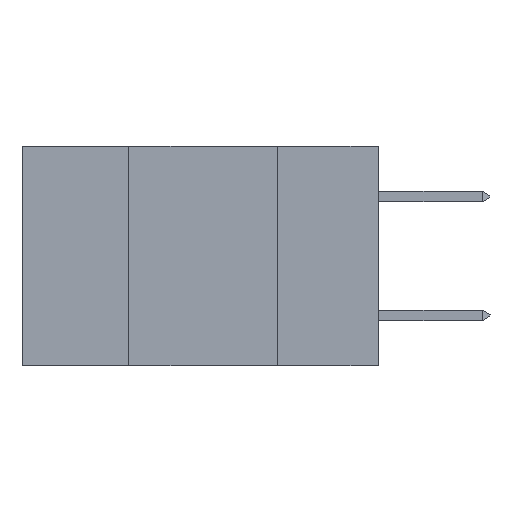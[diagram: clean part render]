
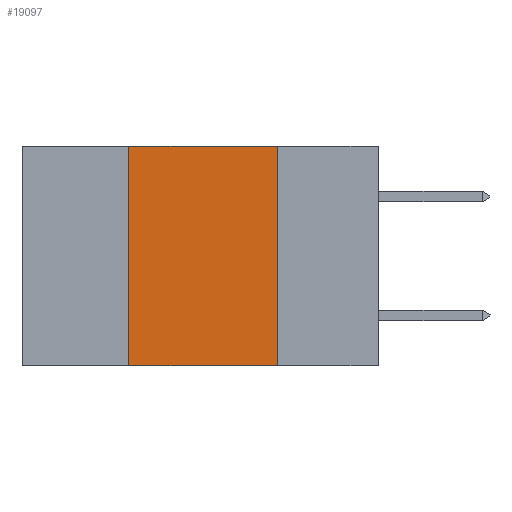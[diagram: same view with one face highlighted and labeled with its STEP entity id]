
A CAD part, left-side view. The second image highlights one B-rep face of the part: STEP entity #19097.
In plain terms, the highlighted planar face has unit normal (-1, 0, 0).
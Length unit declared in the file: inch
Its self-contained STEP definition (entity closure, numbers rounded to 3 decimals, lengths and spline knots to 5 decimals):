
#133 = DIRECTION ( 'NONE',  ( 1., 0., 0. ) ) ;
#151 = DIRECTION ( 'NONE',  ( 0., 0., -1. ) ) ;
#1029 = CARTESIAN_POINT ( 'NONE',  ( 0., 0.17, 0. ) ) ;
#1244 = EDGE_CURVE ( 'NONE', #16846, #17087, #15671, .T. ) ;
#1472 = CARTESIAN_POINT ( 'NONE',  ( 0., 0.42, 0. ) ) ;
#3541 = CARTESIAN_POINT ( 'NONE',  ( 0., 0.6, 0. ) ) ;
#5162 = EDGE_LOOP ( 'NONE', ( #14097, #17059, #18329, #17991 ) ) ;
#5560 = CARTESIAN_POINT ( 'NONE',  ( 0., 0.6, -0.37 ) ) ;
#5833 = DIRECTION ( 'NONE',  ( 0., 0., -1. ) ) ;
#6802 = CARTESIAN_POINT ( 'NONE',  ( 0., 0.42, 0. ) ) ;
#6810 = VERTEX_POINT ( 'NONE', #1029 ) ;
#7404 = PLANE ( 'NONE',  #19030 ) ;
#8198 = LINE ( 'NONE', #3541, #17657 ) ;
#8751 = EDGE_CURVE ( 'NONE', #17087, #6810, #8198, .T. ) ;
#10148 = VECTOR ( 'NONE', #18928, 39.37008 ) ;
#10958 = DIRECTION ( 'NONE',  ( 0., -1., 0. ) ) ;
#11115 = LINE ( 'NONE', #17875, #18042 ) ;
#11229 = EDGE_CURVE ( 'NONE', #6810, #11600, #11115, .T. ) ;
#11600 = VERTEX_POINT ( 'NONE', #17596 ) ;
#12175 = EDGE_CURVE ( 'NONE', #16846, #11600, #12678, .T. ) ;
#12678 = LINE ( 'NONE', #5560, #10148 ) ;
#13256 = CARTESIAN_POINT ( 'NONE',  ( 0., 0.6, 0. ) ) ;
#13940 = FACE_OUTER_BOUND ( 'NONE', #5162, .T. ) ;
#14097 = ORIENTED_EDGE ( 'NONE', *, *, #11229, .F. ) ;
#14977 = VECTOR ( 'NONE', #17121, 39.37008 ) ;
#15671 = LINE ( 'NONE', #6802, #14977 ) ;
#15726 = CARTESIAN_POINT ( 'NONE',  ( 0., 0.42, -0.37 ) ) ;
#16846 = VERTEX_POINT ( 'NONE', #15726 ) ;
#17059 = ORIENTED_EDGE ( 'NONE', *, *, #8751, .F. ) ;
#17087 = VERTEX_POINT ( 'NONE', #1472 ) ;
#17121 = DIRECTION ( 'NONE',  ( 0., 0., 1. ) ) ;
#17596 = CARTESIAN_POINT ( 'NONE',  ( 0., 0.17, -0.37 ) ) ;
#17657 = VECTOR ( 'NONE', #10958, 39.37008 ) ;
#17875 = CARTESIAN_POINT ( 'NONE',  ( 0., 0.17, 0. ) ) ;
#17991 = ORIENTED_EDGE ( 'NONE', *, *, #12175, .T. ) ;
#18042 = VECTOR ( 'NONE', #151, 39.37008 ) ;
#18329 = ORIENTED_EDGE ( 'NONE', *, *, #1244, .F. ) ;
#18928 = DIRECTION ( 'NONE',  ( 0., -1., 0. ) ) ;
#19030 = AXIS2_PLACEMENT_3D ( 'NONE', #13256, #133, #5833 ) ;
#19097 = ADVANCED_FACE ( 'NONE', ( #13940 ), #7404, .F. ) ;
